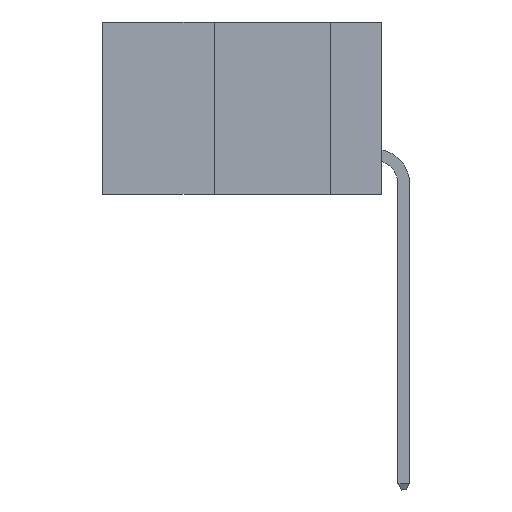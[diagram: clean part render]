
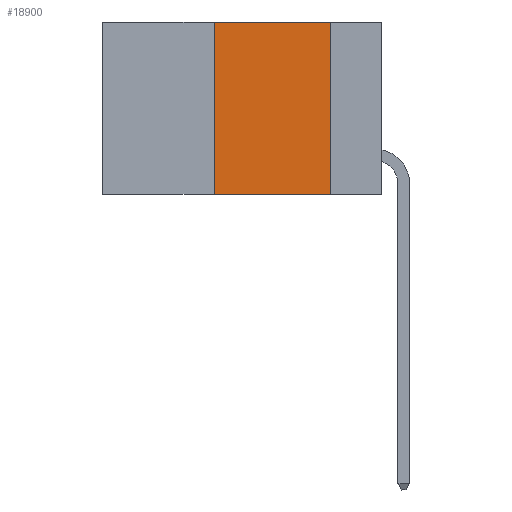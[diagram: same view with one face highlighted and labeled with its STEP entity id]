
A CAD part, left-side view. The second image highlights one B-rep face of the part: STEP entity #18900.
In plain terms, the highlighted planar face has unit normal (-1, 0, 0).
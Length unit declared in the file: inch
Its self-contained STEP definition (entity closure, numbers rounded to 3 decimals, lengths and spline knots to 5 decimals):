
#361 = LINE ( 'NONE', #7397, #19916 ) ;
#749 = CARTESIAN_POINT ( 'NONE',  ( 0., 0.11, -0.37 ) ) ;
#1680 = CARTESIAN_POINT ( 'NONE',  ( 0., 0.6, -0.37 ) ) ;
#3075 = EDGE_CURVE ( 'NONE', #16853, #3128, #17552, .T. ) ;
#3128 = VERTEX_POINT ( 'NONE', #19925 ) ;
#3293 = CARTESIAN_POINT ( 'NONE',  ( 0., 0.6, 0. ) ) ;
#5242 = DIRECTION ( 'NONE',  ( 1., 0., 0. ) ) ;
#5534 = CARTESIAN_POINT ( 'NONE',  ( 0., 0.36, -0.37 ) ) ;
#5810 = AXIS2_PLACEMENT_3D ( 'NONE', #3293, #5242, #18366 ) ;
#6647 = ORIENTED_EDGE ( 'NONE', *, *, #15952, .F. ) ;
#6839 = EDGE_LOOP ( 'NONE', ( #6647, #7845, #22664, #8449 ) ) ;
#7325 = LINE ( 'NONE', #20379, #21593 ) ;
#7397 = CARTESIAN_POINT ( 'NONE',  ( 0., 0.11, 0. ) ) ;
#7600 = VECTOR ( 'NONE', #18536, 39.37008 ) ;
#7771 = VERTEX_POINT ( 'NONE', #5534 ) ;
#7845 = ORIENTED_EDGE ( 'NONE', *, *, #3075, .F. ) ;
#8449 = ORIENTED_EDGE ( 'NONE', *, *, #19627, .T. ) ;
#9389 = DIRECTION ( 'NONE',  ( 0., -1., 0. ) ) ;
#14711 = PLANE ( 'NONE',  #5810 ) ;
#15751 = CARTESIAN_POINT ( 'NONE',  ( 0., 0.36, 0. ) ) ;
#15801 = FACE_OUTER_BOUND ( 'NONE', #6839, .T. ) ;
#15952 = EDGE_CURVE ( 'NONE', #3128, #19350, #361, .T. ) ;
#16853 = VERTEX_POINT ( 'NONE', #15751 ) ;
#17182 = EDGE_CURVE ( 'NONE', #7771, #16853, #7325, .T. ) ;
#17536 = CARTESIAN_POINT ( 'NONE',  ( 0., 0.6, 0. ) ) ;
#17552 = LINE ( 'NONE', #17536, #7600 ) ;
#18366 = DIRECTION ( 'NONE',  ( 0., 0., -1. ) ) ;
#18536 = DIRECTION ( 'NONE',  ( 0., -1., 0. ) ) ;
#18577 = DIRECTION ( 'NONE',  ( 0., 0., -1. ) ) ;
#18900 = ADVANCED_FACE ( 'NONE', ( #15801 ), #14711, .F. ) ;
#19339 = VECTOR ( 'NONE', #9389, 39.37008 ) ;
#19350 = VERTEX_POINT ( 'NONE', #749 ) ;
#19627 = EDGE_CURVE ( 'NONE', #7771, #19350, #19911, .T. ) ;
#19911 = LINE ( 'NONE', #1680, #19339 ) ;
#19916 = VECTOR ( 'NONE', #18577, 39.37008 ) ;
#19925 = CARTESIAN_POINT ( 'NONE',  ( 0., 0.11, 0. ) ) ;
#20379 = CARTESIAN_POINT ( 'NONE',  ( 0., 0.36, 0. ) ) ;
#21593 = VECTOR ( 'NONE', #24072, 39.37008 ) ;
#22664 = ORIENTED_EDGE ( 'NONE', *, *, #17182, .F. ) ;
#24072 = DIRECTION ( 'NONE',  ( 0., 0., 1. ) ) ;
